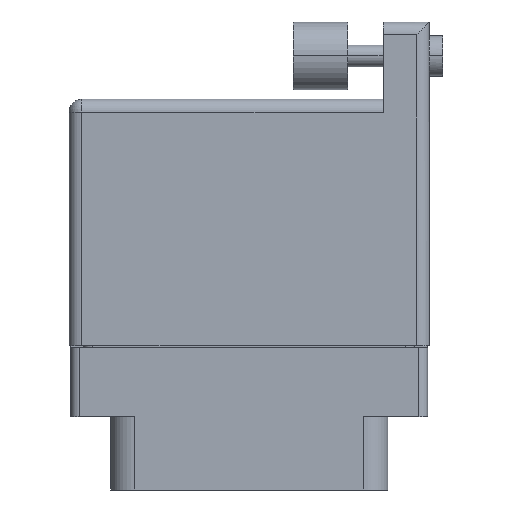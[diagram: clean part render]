
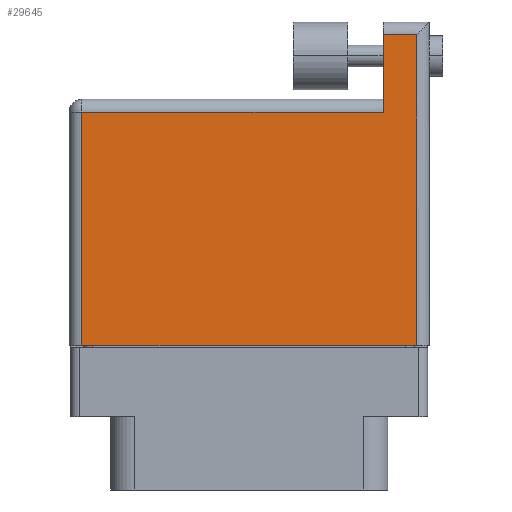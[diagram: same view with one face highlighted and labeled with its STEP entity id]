
A CAD part, front view. The second image highlights one B-rep face of the part: STEP entity #29645.
In plain terms, the highlighted face is planar.
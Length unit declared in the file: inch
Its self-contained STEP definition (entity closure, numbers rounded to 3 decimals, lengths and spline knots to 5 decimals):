
#241 = VERTEX_POINT ( 'NONE', #13711 ) ;
#441 = DIRECTION ( 'NONE',  ( -1., 0., 0. ) ) ;
#3632 = EDGE_CURVE ( 'NONE', #24167, #18321, #15333, .T. ) ;
#3869 = CARTESIAN_POINT ( 'NONE',  ( 0.4925, 1.043, 0.3575 ) ) ;
#4437 = LINE ( 'NONE', #21765, #28768 ) ;
#5463 = CARTESIAN_POINT ( 'NONE',  ( 0.6155, 1.043, 0.3575 ) ) ;
#5730 = VECTOR ( 'NONE', #8417, 39.37008 ) ;
#7464 = CARTESIAN_POINT ( 'NONE',  ( -0.6625, 0.759, 0.3575 ) ) ;
#7643 = DIRECTION ( 'NONE',  ( 0., -1., 0. ) ) ;
#7868 = VECTOR ( 'NONE', #27730, 39.37008 ) ;
#8417 = DIRECTION ( 'NONE',  ( -1., 0., 0. ) ) ;
#8479 = VERTEX_POINT ( 'NONE', #17455 ) ;
#9633 = CARTESIAN_POINT ( 'NONE',  ( -0.6625, 0.806, 0.3575 ) ) ;
#9671 = ORIENTED_EDGE ( 'NONE', *, *, #14742, .T. ) ;
#9786 = VECTOR ( 'NONE', #441, 39.37008 ) ;
#10057 = LINE ( 'NONE', #12012, #13364 ) ;
#10197 = LINE ( 'NONE', #23247, #10931 ) ;
#10499 = EDGE_CURVE ( 'NONE', #14449, #24167, #24466, .T. ) ;
#10931 = VECTOR ( 'NONE', #27973, 39.37008 ) ;
#11202 = ORIENTED_EDGE ( 'NONE', *, *, #21335, .T. ) ;
#11723 = PLANE ( 'NONE',  #21899 ) ;
#12012 = CARTESIAN_POINT ( 'NONE',  ( 0.6155, 1.09, 0.3575 ) ) ;
#12373 = ORIENTED_EDGE ( 'NONE', *, *, #27780, .T. ) ;
#13211 = CARTESIAN_POINT ( 'NONE',  ( 0.4925, 1.09, 0.3575 ) ) ;
#13364 = VECTOR ( 'NONE', #23651, 39.37008 ) ;
#13479 = LINE ( 'NONE', #3869, #5730 ) ;
#13711 = CARTESIAN_POINT ( 'NONE',  ( 0.6155, -0.1, 0.3575 ) ) ;
#13892 = DIRECTION ( 'NONE',  ( -1., 0., 0. ) ) ;
#14067 = DIRECTION ( 'NONE',  ( 0., 0., -1. ) ) ;
#14449 = VERTEX_POINT ( 'NONE', #17722 ) ;
#14528 = ORIENTED_EDGE ( 'NONE', *, *, #3632, .T. ) ;
#14742 = EDGE_CURVE ( 'NONE', #241, #24386, #10057, .T. ) ;
#15333 = LINE ( 'NONE', #7464, #9786 ) ;
#15957 = EDGE_LOOP ( 'NONE', ( #25249, #9671, #11202, #22761, #14528, #12373 ) ) ;
#17455 = CARTESIAN_POINT ( 'NONE',  ( -0.6155, -0.1, 0.3575 ) ) ;
#17722 = CARTESIAN_POINT ( 'NONE',  ( 0.4925, 1.043, 0.3575 ) ) ;
#18321 = VERTEX_POINT ( 'NONE', #19592 ) ;
#19592 = CARTESIAN_POINT ( 'NONE',  ( -0.6155, 0.759, 0.3575 ) ) ;
#21335 = EDGE_CURVE ( 'NONE', #24386, #14449, #13479, .T. ) ;
#21765 = CARTESIAN_POINT ( 'NONE',  ( -0.6155, -0.1, 0.3575 ) ) ;
#21899 = AXIS2_PLACEMENT_3D ( 'NONE', #9633, #14067, #13892 ) ;
#22761 = ORIENTED_EDGE ( 'NONE', *, *, #10499, .T. ) ;
#23247 = CARTESIAN_POINT ( 'NONE',  ( -0.6625, -0.1, 0.3575 ) ) ;
#23615 = EDGE_CURVE ( 'NONE', #8479, #241, #10197, .T. ) ;
#23651 = DIRECTION ( 'NONE',  ( 0., 1., 0. ) ) ;
#24167 = VERTEX_POINT ( 'NONE', #25478 ) ;
#24386 = VERTEX_POINT ( 'NONE', #5463 ) ;
#24466 = LINE ( 'NONE', #13211, #7868 ) ;
#25249 = ORIENTED_EDGE ( 'NONE', *, *, #23615, .T. ) ;
#25478 = CARTESIAN_POINT ( 'NONE',  ( 0.4925, 0.759, 0.3575 ) ) ;
#26067 = FACE_OUTER_BOUND ( 'NONE', #15957, .T. ) ;
#27730 = DIRECTION ( 'NONE',  ( 0., -1., 0. ) ) ;
#27780 = EDGE_CURVE ( 'NONE', #18321, #8479, #4437, .T. ) ;
#27973 = DIRECTION ( 'NONE',  ( 1., 0., 0. ) ) ;
#28768 = VECTOR ( 'NONE', #7643, 39.37008 ) ;
#29645 = ADVANCED_FACE ( 'NONE', ( #26067 ), #11723, .F. ) ;
